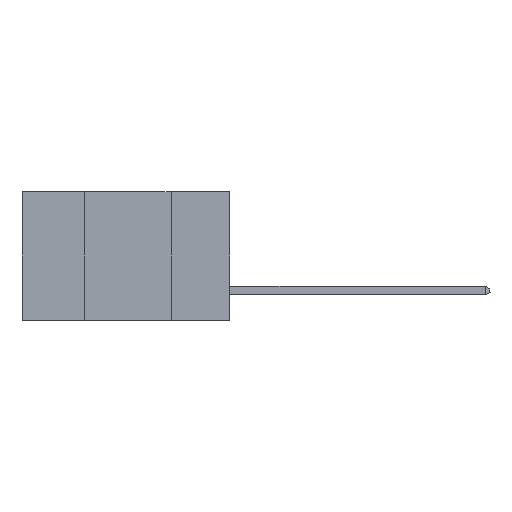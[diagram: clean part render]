
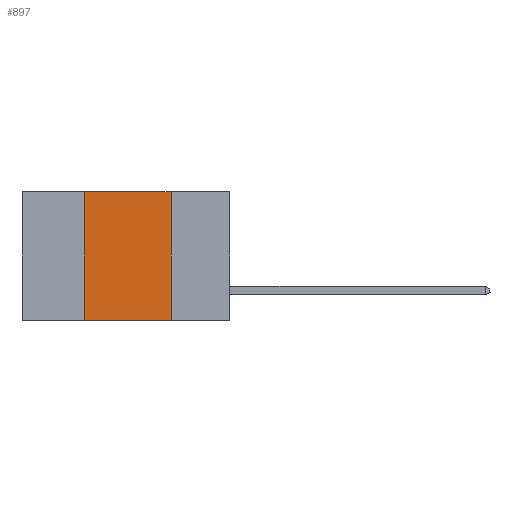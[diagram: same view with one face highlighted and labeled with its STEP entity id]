
A CAD part, left-side view. The second image highlights one B-rep face of the part: STEP entity #897.
In plain terms, the highlighted planar face has unit normal (-1, 0, 0).
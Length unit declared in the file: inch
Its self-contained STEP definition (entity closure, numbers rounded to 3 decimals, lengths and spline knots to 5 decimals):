
#532 = DIRECTION ( 'NONE',  ( 0., 0., 1. ) ) ;
#871 = CARTESIAN_POINT ( 'NONE',  ( 0., 0.42, -0.37 ) ) ;
#897 = ADVANCED_FACE ( 'NONE', ( #12822 ), #10264, .F. ) ;
#1518 = LINE ( 'NONE', #10903, #4080 ) ;
#1695 = LINE ( 'NONE', #18582, #20237 ) ;
#3895 = ORIENTED_EDGE ( 'NONE', *, *, #11889, .F. ) ;
#4080 = VECTOR ( 'NONE', #20303, 39.37008 ) ;
#4488 = DIRECTION ( 'NONE',  ( 0., -1., 0. ) ) ;
#5286 = DIRECTION ( 'NONE',  ( 1., 0., 0. ) ) ;
#6420 = LINE ( 'NONE', #10060, #12110 ) ;
#6549 = EDGE_CURVE ( 'NONE', #12555, #9476, #17684, .T. ) ;
#9476 = VERTEX_POINT ( 'NONE', #21343 ) ;
#10016 = ORIENTED_EDGE ( 'NONE', *, *, #14248, .F. ) ;
#10060 = CARTESIAN_POINT ( 'NONE',  ( 0., 0.17, 0. ) ) ;
#10109 = ORIENTED_EDGE ( 'NONE', *, *, #13985, .F. ) ;
#10125 = DIRECTION ( 'NONE',  ( 0., 0., -1. ) ) ;
#10179 = CARTESIAN_POINT ( 'NONE',  ( 0., 0.17, 0. ) ) ;
#10264 = PLANE ( 'NONE',  #15948 ) ;
#10400 = CARTESIAN_POINT ( 'NONE',  ( 0., 0.6, 0. ) ) ;
#10903 = CARTESIAN_POINT ( 'NONE',  ( 0., 0.6, 0. ) ) ;
#11889 = EDGE_CURVE ( 'NONE', #20054, #19157, #1518, .T. ) ;
#12110 = VECTOR ( 'NONE', #10125, 39.37008 ) ;
#12555 = VERTEX_POINT ( 'NONE', #871 ) ;
#12822 = FACE_OUTER_BOUND ( 'NONE', #19317, .T. ) ;
#13330 = VECTOR ( 'NONE', #4488, 39.37008 ) ;
#13658 = CARTESIAN_POINT ( 'NONE',  ( 0., 0.42, 0. ) ) ;
#13985 = EDGE_CURVE ( 'NONE', #19157, #9476, #6420, .T. ) ;
#14248 = EDGE_CURVE ( 'NONE', #12555, #20054, #1695, .T. ) ;
#14453 = CARTESIAN_POINT ( 'NONE',  ( 0., 0.6, -0.37 ) ) ;
#15456 = DIRECTION ( 'NONE',  ( 0., 0., -1. ) ) ;
#15948 = AXIS2_PLACEMENT_3D ( 'NONE', #10400, #5286, #15456 ) ;
#17684 = LINE ( 'NONE', #14453, #13330 ) ;
#18582 = CARTESIAN_POINT ( 'NONE',  ( 0., 0.42, 0. ) ) ;
#19157 = VERTEX_POINT ( 'NONE', #10179 ) ;
#19317 = EDGE_LOOP ( 'NONE', ( #10109, #3895, #10016, #20482 ) ) ;
#20054 = VERTEX_POINT ( 'NONE', #13658 ) ;
#20237 = VECTOR ( 'NONE', #532, 39.37008 ) ;
#20303 = DIRECTION ( 'NONE',  ( 0., -1., 0. ) ) ;
#20482 = ORIENTED_EDGE ( 'NONE', *, *, #6549, .T. ) ;
#21343 = CARTESIAN_POINT ( 'NONE',  ( 0., 0.17, -0.37 ) ) ;
